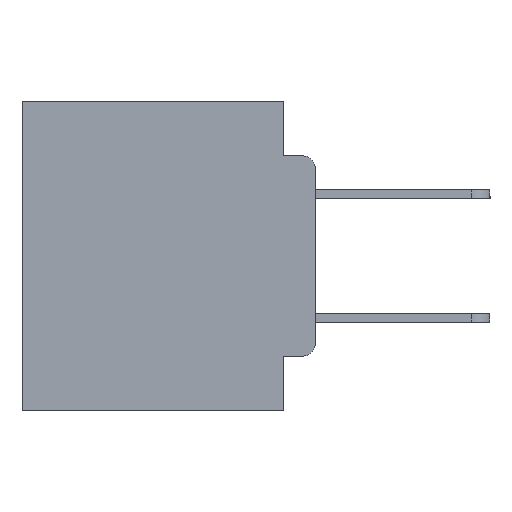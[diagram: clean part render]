
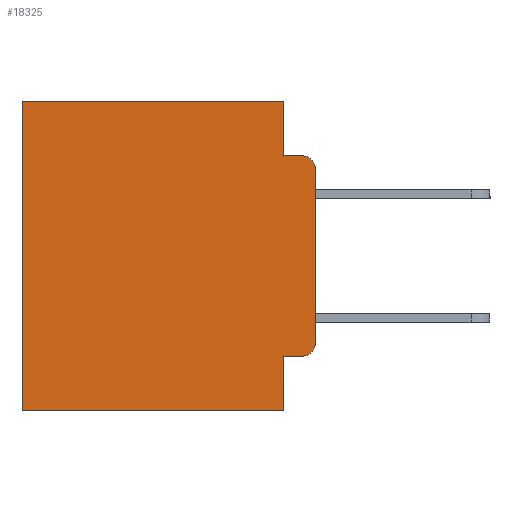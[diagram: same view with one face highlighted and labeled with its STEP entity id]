
A CAD part, left-side view. The second image highlights one B-rep face of the part: STEP entity #18325.
In plain terms, the highlighted planar face has unit normal (-1, 0, 0).
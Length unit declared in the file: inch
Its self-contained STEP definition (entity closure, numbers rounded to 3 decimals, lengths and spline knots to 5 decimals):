
#471 = EDGE_CURVE ( 'NONE', #24864, #18596, #25482, .T. ) ;
#565 = CARTESIAN_POINT ( 'NONE',  ( 0.298, 0.051, 0. ) ) ;
#604 = CARTESIAN_POINT ( 'NONE',  ( 0.298, 0., 0. ) ) ;
#988 = VECTOR ( 'NONE', #17728, 39.37008 ) ;
#1998 = ORIENTED_EDGE ( 'NONE', *, *, #13004, .F. ) ;
#2171 = VERTEX_POINT ( 'NONE', #12660 ) ;
#2199 = VECTOR ( 'NONE', #15309, 39.37008 ) ;
#2289 = VECTOR ( 'NONE', #18355, 39.37008 ) ;
#3076 = VERTEX_POINT ( 'NONE', #9761 ) ;
#3284 = EDGE_CURVE ( 'NONE', #3076, #24864, #18157, .T. ) ;
#3636 = VERTEX_POINT ( 'NONE', #10310 ) ;
#3956 = CARTESIAN_POINT ( 'NONE',  ( 0.298, 0., 0. ) ) ;
#4219 = LINE ( 'NONE', #9349, #15180 ) ;
#4727 = EDGE_CURVE ( 'NONE', #3076, #7346, #4948, .T. ) ;
#4948 = LINE ( 'NONE', #565, #24188 ) ;
#5086 = VERTEX_POINT ( 'NONE', #10077 ) ;
#5233 = CARTESIAN_POINT ( 'NONE',  ( 0.298, 0.02, -0.1085 ) ) ;
#5435 = CARTESIAN_POINT ( 'NONE',  ( 0.298, 0.051, 0. ) ) ;
#6117 = EDGE_CURVE ( 'NONE', #5086, #15779, #23450, .T. ) ;
#6123 = DIRECTION ( 'NONE',  ( 0., -1., 0. ) ) ;
#6866 = VERTEX_POINT ( 'NONE', #7482 ) ;
#6955 = DIRECTION ( 'NONE',  ( 1., 0., 0. ) ) ;
#7197 = LINE ( 'NONE', #19787, #16833 ) ;
#7319 = DIRECTION ( 'NONE',  ( 0., 0., -1. ) ) ;
#7346 = VERTEX_POINT ( 'NONE', #13003 ) ;
#7482 = CARTESIAN_POINT ( 'NONE',  ( 0.298, 0.051, -0.0885 ) ) ;
#9256 = ORIENTED_EDGE ( 'NONE', *, *, #13718, .T. ) ;
#9349 = CARTESIAN_POINT ( 'NONE',  ( 0.298, 0., 0. ) ) ;
#9658 = CARTESIAN_POINT ( 'NONE',  ( 0.298, 0.02, -0.3915 ) ) ;
#9761 = CARTESIAN_POINT ( 'NONE',  ( 0.298, 0.051, -0.4115 ) ) ;
#10077 = CARTESIAN_POINT ( 'NONE',  ( 0.298, 0.473, 0. ) ) ;
#10310 = CARTESIAN_POINT ( 'NONE',  ( 0.298, 0.051, 0. ) ) ;
#10314 = ORIENTED_EDGE ( 'NONE', *, *, #19836, .F. ) ;
#10955 = ORIENTED_EDGE ( 'NONE', *, *, #4727, .F. ) ;
#11539 = AXIS2_PLACEMENT_3D ( 'NONE', #9658, #20838, #18154 ) ;
#11649 = EDGE_CURVE ( 'NONE', #3636, #6866, #12093, .T. ) ;
#11689 = VERTEX_POINT ( 'NONE', #15872 ) ;
#12093 = LINE ( 'NONE', #5435, #988 ) ;
#12643 = VECTOR ( 'NONE', #14812, 39.37008 ) ;
#12660 = CARTESIAN_POINT ( 'NONE',  ( 0.298, 0., -0.1085 ) ) ;
#13003 = CARTESIAN_POINT ( 'NONE',  ( 0.298, 0.051, -0.5 ) ) ;
#13004 = EDGE_CURVE ( 'NONE', #6866, #11689, #7197, .T. ) ;
#13295 = LINE ( 'NONE', #3956, #2289 ) ;
#13353 = EDGE_CURVE ( 'NONE', #7346, #15779, #18060, .T. ) ;
#13368 = AXIS2_PLACEMENT_3D ( 'NONE', #604, #6955, #21276 ) ;
#13718 = EDGE_CURVE ( 'NONE', #3636, #5086, #4219, .T. ) ;
#13893 = CARTESIAN_POINT ( 'NONE',  ( 0.298, 0.473, -0.5 ) ) ;
#13945 = ORIENTED_EDGE ( 'NONE', *, *, #6117, .T. ) ;
#14037 = CARTESIAN_POINT ( 'NONE',  ( 0.298, 0., -0.3915 ) ) ;
#14400 = EDGE_CURVE ( 'NONE', #2171, #11689, #22175, .T. ) ;
#14812 = DIRECTION ( 'NONE',  ( 0., 1., 0. ) ) ;
#15180 = VECTOR ( 'NONE', #23633, 39.37008 ) ;
#15309 = DIRECTION ( 'NONE',  ( 0., 0., -1. ) ) ;
#15779 = VERTEX_POINT ( 'NONE', #13893 ) ;
#15872 = CARTESIAN_POINT ( 'NONE',  ( 0.298, 0.02, -0.0885 ) ) ;
#16552 = ORIENTED_EDGE ( 'NONE', *, *, #13353, .F. ) ;
#16833 = VECTOR ( 'NONE', #23839, 39.37008 ) ;
#16869 = CARTESIAN_POINT ( 'NONE',  ( 0.298, 0., -0.5 ) ) ;
#17728 = DIRECTION ( 'NONE',  ( 0., 0., -1. ) ) ;
#18060 = LINE ( 'NONE', #16869, #12643 ) ;
#18104 = ORIENTED_EDGE ( 'NONE', *, *, #3284, .T. ) ;
#18154 = DIRECTION ( 'NONE',  ( 0., 0., -1. ) ) ;
#18157 = LINE ( 'NONE', #23523, #24263 ) ;
#18325 = ADVANCED_FACE ( 'NONE', ( #22021 ), #19196, .F. ) ;
#18355 = DIRECTION ( 'NONE',  ( 0., 0., -1. ) ) ;
#18596 = VERTEX_POINT ( 'NONE', #14037 ) ;
#19196 = PLANE ( 'NONE',  #13368 ) ;
#19549 = DIRECTION ( 'NONE',  ( -1., 0., 0. ) ) ;
#19787 = CARTESIAN_POINT ( 'NONE',  ( 0.298, 0.051, -0.0885 ) ) ;
#19836 = EDGE_CURVE ( 'NONE', #2171, #18596, #13295, .T. ) ;
#20838 = DIRECTION ( 'NONE',  ( -1., 0., 0. ) ) ;
#21276 = DIRECTION ( 'NONE',  ( 0., 0., -1. ) ) ;
#21462 = CARTESIAN_POINT ( 'NONE',  ( 0.298, 0.473, 0. ) ) ;
#22021 = FACE_OUTER_BOUND ( 'NONE', #26482, .T. ) ;
#22175 = CIRCLE ( 'NONE', #24122, 0.02 ) ;
#22442 = ORIENTED_EDGE ( 'NONE', *, *, #14400, .T. ) ;
#23450 = LINE ( 'NONE', #21462, #2199 ) ;
#23523 = CARTESIAN_POINT ( 'NONE',  ( 0.298, 0.051, -0.4115 ) ) ;
#23633 = DIRECTION ( 'NONE',  ( 0., 1., 0. ) ) ;
#23812 = ORIENTED_EDGE ( 'NONE', *, *, #11649, .F. ) ;
#23839 = DIRECTION ( 'NONE',  ( 0., -1., 0. ) ) ;
#24122 = AXIS2_PLACEMENT_3D ( 'NONE', #5233, #19549, #7319 ) ;
#24188 = VECTOR ( 'NONE', #26540, 39.37008 ) ;
#24207 = ORIENTED_EDGE ( 'NONE', *, *, #471, .T. ) ;
#24263 = VECTOR ( 'NONE', #6123, 39.37008 ) ;
#24864 = VERTEX_POINT ( 'NONE', #25478 ) ;
#25478 = CARTESIAN_POINT ( 'NONE',  ( 0.298, 0.02, -0.4115 ) ) ;
#25482 = CIRCLE ( 'NONE', #11539, 0.02 ) ;
#26482 = EDGE_LOOP ( 'NONE', ( #10314, #22442, #1998, #23812, #9256, #13945, #16552, #10955, #18104, #24207 ) ) ;
#26540 = DIRECTION ( 'NONE',  ( 0., 0., -1. ) ) ;
